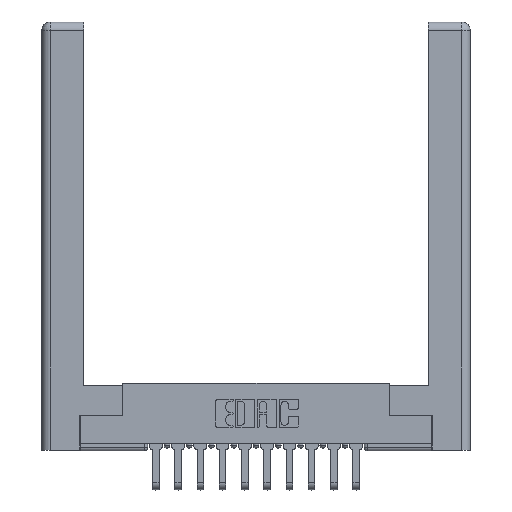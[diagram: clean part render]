
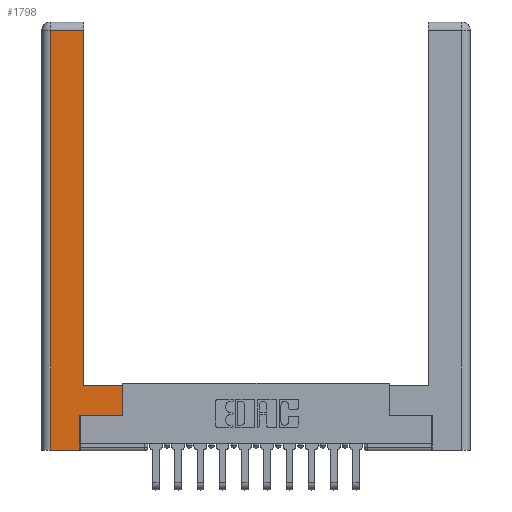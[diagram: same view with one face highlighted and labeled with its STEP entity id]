
A CAD part, top view. The second image highlights one B-rep face of the part: STEP entity #1798.
In plain terms, the highlighted planar face has unit normal (0, 0, 1).
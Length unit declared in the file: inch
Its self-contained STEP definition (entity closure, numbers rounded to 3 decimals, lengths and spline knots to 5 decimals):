
#208 = CARTESIAN_POINT ( 'NONE',  ( 0.0615, 0., 0. ) ) ;
#440 = DIRECTION ( 'NONE',  ( 0., 1., 0. ) ) ;
#653 = ORIENTED_EDGE ( 'NONE', *, *, #11186, .T. ) ;
#933 = DIRECTION ( 'NONE',  ( 0., -1., 0. ) ) ;
#1009 = PLANE ( 'NONE',  #5617 ) ;
#1139 = ORIENTED_EDGE ( 'NONE', *, *, #4053, .T. ) ;
#1425 = CARTESIAN_POINT ( 'NONE',  ( 0.295, 2.94, 0. ) ) ;
#1439 = VERTEX_POINT ( 'NONE', #13146 ) ;
#1545 = DIRECTION ( 'NONE',  ( 0., 1., 0. ) ) ;
#1706 = DIRECTION ( 'NONE',  ( -1., 0., 0. ) ) ;
#1724 = VERTEX_POINT ( 'NONE', #6496 ) ;
#1798 = ADVANCED_FACE ( 'NONE', ( #2561 ), #1009, .F. ) ;
#1914 = EDGE_CURVE ( 'NONE', #11757, #9835, #10888, .T. ) ;
#2002 = CARTESIAN_POINT ( 'NONE',  ( 0.565, 0.245, 0. ) ) ;
#2084 = DIRECTION ( 'NONE',  ( 0., 0., -1. ) ) ;
#2159 = CARTESIAN_POINT ( 'NONE',  ( 0.0615, 0., 0. ) ) ;
#2281 = DIRECTION ( 'NONE',  ( 0., 1., 0. ) ) ;
#2561 = FACE_OUTER_BOUND ( 'NONE', #12976, .T. ) ;
#2646 = VECTOR ( 'NONE', #10863, 39.37008 ) ;
#2833 = CARTESIAN_POINT ( 'NONE',  ( 0.0615, 2.94, 0. ) ) ;
#3330 = VERTEX_POINT ( 'NONE', #208 ) ;
#3359 = DIRECTION ( 'NONE',  ( -1., 0., 0. ) ) ;
#3570 = VECTOR ( 'NONE', #5006, 39.37008 ) ;
#4053 = EDGE_CURVE ( 'NONE', #13595, #12069, #4523, .T. ) ;
#4396 = CARTESIAN_POINT ( 'NONE',  ( 0., 0., 0. ) ) ;
#4523 = LINE ( 'NONE', #11004, #7114 ) ;
#5006 = DIRECTION ( 'NONE',  ( 1., 0., 0. ) ) ;
#5105 = CARTESIAN_POINT ( 'NONE',  ( 0.265, 0., 0. ) ) ;
#5160 = CARTESIAN_POINT ( 'NONE',  ( 0.265, 0.245, 0. ) ) ;
#5260 = VERTEX_POINT ( 'NONE', #13194 ) ;
#5617 = AXIS2_PLACEMENT_3D ( 'NONE', #4396, #2084, #3359 ) ;
#5632 = DIRECTION ( 'NONE',  ( 1., 0., 0. ) ) ;
#5859 = LINE ( 'NONE', #2833, #9175 ) ;
#5973 = CARTESIAN_POINT ( 'NONE',  ( 0.295, 0.45, 0. ) ) ;
#6457 = VECTOR ( 'NONE', #933, 39.37008 ) ;
#6463 = ORIENTED_EDGE ( 'NONE', *, *, #12675, .T. ) ;
#6496 = CARTESIAN_POINT ( 'NONE',  ( 0.0615, 2.94, 0. ) ) ;
#6668 = CARTESIAN_POINT ( 'NONE',  ( 0.565, 0.245, 0. ) ) ;
#6673 = ORIENTED_EDGE ( 'NONE', *, *, #10723, .T. ) ;
#6732 = LINE ( 'NONE', #5105, #3570 ) ;
#7114 = VECTOR ( 'NONE', #440, 39.37008 ) ;
#8983 = VECTOR ( 'NONE', #1545, 39.37008 ) ;
#9028 = EDGE_CURVE ( 'NONE', #1439, #13595, #12508, .T. ) ;
#9109 = EDGE_CURVE ( 'NONE', #1724, #3330, #9396, .T. ) ;
#9175 = VECTOR ( 'NONE', #1706, 39.37008 ) ;
#9396 = LINE ( 'NONE', #2159, #6457 ) ;
#9588 = CARTESIAN_POINT ( 'NONE',  ( 0.295, 0.45, 0. ) ) ;
#9614 = VECTOR ( 'NONE', #2281, 39.37008 ) ;
#9627 = ORIENTED_EDGE ( 'NONE', *, *, #9028, .T. ) ;
#9709 = CARTESIAN_POINT ( 'NONE',  ( 0.565, 0.45, 0. ) ) ;
#9766 = VECTOR ( 'NONE', #5632, 39.37008 ) ;
#9835 = VERTEX_POINT ( 'NONE', #1425 ) ;
#10221 = LINE ( 'NONE', #5973, #2646 ) ;
#10582 = ORIENTED_EDGE ( 'NONE', *, *, #1914, .T. ) ;
#10723 = EDGE_CURVE ( 'NONE', #9835, #1724, #5859, .T. ) ;
#10863 = DIRECTION ( 'NONE',  ( -1., 0., 0. ) ) ;
#10888 = LINE ( 'NONE', #14207, #9614 ) ;
#11004 = CARTESIAN_POINT ( 'NONE',  ( 0.565, 0.45, 0. ) ) ;
#11186 = EDGE_CURVE ( 'NONE', #5260, #1439, #13762, .T. ) ;
#11757 = VERTEX_POINT ( 'NONE', #9588 ) ;
#12069 = VERTEX_POINT ( 'NONE', #9709 ) ;
#12104 = ORIENTED_EDGE ( 'NONE', *, *, #9109, .T. ) ;
#12129 = EDGE_CURVE ( 'NONE', #3330, #5260, #6732, .T. ) ;
#12508 = LINE ( 'NONE', #6668, #9766 ) ;
#12675 = EDGE_CURVE ( 'NONE', #12069, #11757, #10221, .T. ) ;
#12976 = EDGE_LOOP ( 'NONE', ( #10582, #6673, #12104, #13057, #653, #9627, #1139, #6463 ) ) ;
#13057 = ORIENTED_EDGE ( 'NONE', *, *, #12129, .T. ) ;
#13146 = CARTESIAN_POINT ( 'NONE',  ( 0.265, 0.245, 0. ) ) ;
#13194 = CARTESIAN_POINT ( 'NONE',  ( 0.265, 0., 0. ) ) ;
#13595 = VERTEX_POINT ( 'NONE', #2002 ) ;
#13762 = LINE ( 'NONE', #5160, #8983 ) ;
#14207 = CARTESIAN_POINT ( 'NONE',  ( 0.295, 3., 0. ) ) ;
